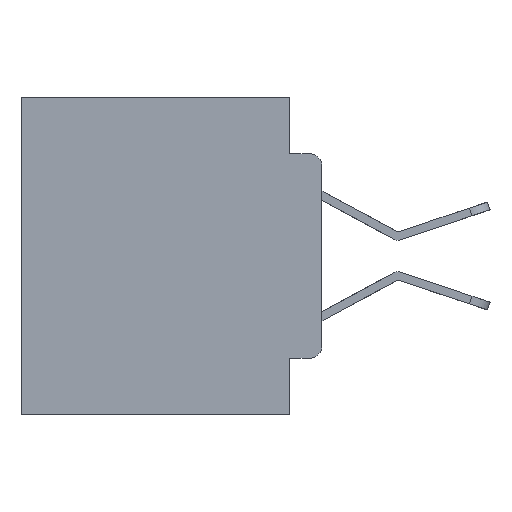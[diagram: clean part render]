
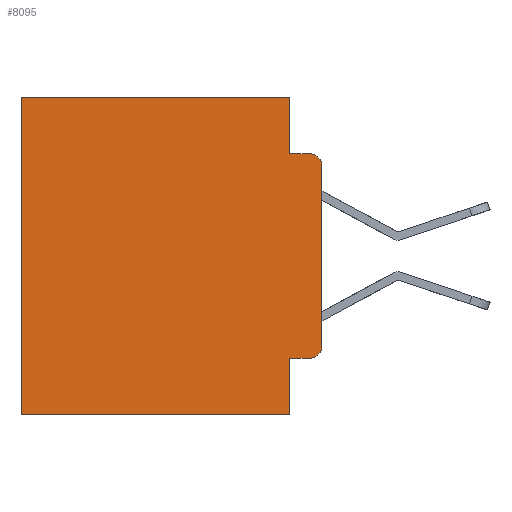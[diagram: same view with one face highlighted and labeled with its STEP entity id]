
A CAD part, left-side view. The second image highlights one B-rep face of the part: STEP entity #8095.
In plain terms, the highlighted planar face has unit normal (-1, 0, 0).
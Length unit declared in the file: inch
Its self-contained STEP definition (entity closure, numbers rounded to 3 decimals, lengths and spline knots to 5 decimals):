
#182 = LINE ( 'NONE', #26400, #10957 ) ;
#1170 = LINE ( 'NONE', #9637, #17663 ) ;
#1172 = AXIS2_PLACEMENT_3D ( 'NONE', #19801, #6941, #21983 ) ;
#1191 = ORIENTED_EDGE ( 'NONE', *, *, #9196, .T. ) ;
#1548 = CARTESIAN_POINT ( 'NONE',  ( 0.298, 0., -0.1085 ) ) ;
#1922 = ORIENTED_EDGE ( 'NONE', *, *, #22513, .T. ) ;
#2360 = CIRCLE ( 'NONE', #20978, 0.02 ) ;
#2890 = LINE ( 'NONE', #6590, #23682 ) ;
#3070 = CARTESIAN_POINT ( 'NONE',  ( 0.298, 0.02, -0.0885 ) ) ;
#3256 = ORIENTED_EDGE ( 'NONE', *, *, #19504, .F. ) ;
#4125 = VERTEX_POINT ( 'NONE', #3070 ) ;
#4140 = DIRECTION ( 'NONE',  ( 0., 0., -1. ) ) ;
#4175 = DIRECTION ( 'NONE',  ( 1., 0., 0. ) ) ;
#4200 = PLANE ( 'NONE',  #6270 ) ;
#4271 = CARTESIAN_POINT ( 'NONE',  ( 0.298, 0., 0. ) ) ;
#4449 = CARTESIAN_POINT ( 'NONE',  ( 0.298, 0., -0.5 ) ) ;
#5339 = LINE ( 'NONE', #4449, #16115 ) ;
#6270 = AXIS2_PLACEMENT_3D ( 'NONE', #4271, #4175, #4140 ) ;
#6590 = CARTESIAN_POINT ( 'NONE',  ( 0.298, 0.051, 0. ) ) ;
#6594 = DIRECTION ( 'NONE',  ( 0., 1., 0. ) ) ;
#6851 = LINE ( 'NONE', #12480, #11910 ) ;
#6941 = DIRECTION ( 'NONE',  ( -1., 0., 0. ) ) ;
#6955 = EDGE_CURVE ( 'NONE', #16703, #4125, #26650, .T. ) ;
#6989 = DIRECTION ( 'NONE',  ( 0., 0., -1. ) ) ;
#7127 = CARTESIAN_POINT ( 'NONE',  ( 0.298, 0.473, -0.5 ) ) ;
#7207 = VERTEX_POINT ( 'NONE', #1548 ) ;
#7759 = DIRECTION ( 'NONE',  ( 0., -1., 0. ) ) ;
#7865 = CARTESIAN_POINT ( 'NONE',  ( 0.298, 0.051, -0.0885 ) ) ;
#7991 = ORIENTED_EDGE ( 'NONE', *, *, #8531, .T. ) ;
#8095 = ADVANCED_FACE ( 'NONE', ( #16720 ), #4200, .F. ) ;
#8531 = EDGE_CURVE ( 'NONE', #12215, #14233, #182, .T. ) ;
#8668 = CARTESIAN_POINT ( 'NONE',  ( 0.298, 0., 0. ) ) ;
#9196 = EDGE_CURVE ( 'NONE', #25642, #13427, #1170, .T. ) ;
#9376 = DIRECTION ( 'NONE',  ( 0., -1., 0. ) ) ;
#9544 = CARTESIAN_POINT ( 'NONE',  ( 0.298, 0.02, -0.1085 ) ) ;
#9637 = CARTESIAN_POINT ( 'NONE',  ( 0.298, 0.473, 0. ) ) ;
#9682 = VECTOR ( 'NONE', #7759, 39.37008 ) ;
#10220 = VECTOR ( 'NONE', #6989, 39.37008 ) ;
#10723 = CARTESIAN_POINT ( 'NONE',  ( 0.298, 0.051, -0.5 ) ) ;
#10957 = VECTOR ( 'NONE', #9376, 39.37008 ) ;
#11684 = DIRECTION ( 'NONE',  ( 0., 0., -1. ) ) ;
#11910 = VECTOR ( 'NONE', #21038, 39.37008 ) ;
#11954 = CARTESIAN_POINT ( 'NONE',  ( 0.298, 0., -0.3915 ) ) ;
#12215 = VERTEX_POINT ( 'NONE', #22609 ) ;
#12480 = CARTESIAN_POINT ( 'NONE',  ( 0.298, 0.051, 0. ) ) ;
#12506 = EDGE_LOOP ( 'NONE', ( #21894, #1922, #16373, #13661, #18630, #1191, #26623, #3256, #7991, #26416 ) ) ;
#13203 = EDGE_CURVE ( 'NONE', #21087, #25642, #22472, .T. ) ;
#13208 = EDGE_CURVE ( 'NONE', #22896, #13427, #5339, .T. ) ;
#13385 = CARTESIAN_POINT ( 'NONE',  ( 0.298, 0.051, 0. ) ) ;
#13427 = VERTEX_POINT ( 'NONE', #7127 ) ;
#13513 = CARTESIAN_POINT ( 'NONE',  ( 0.298, 0., 0. ) ) ;
#13661 = ORIENTED_EDGE ( 'NONE', *, *, #15697, .F. ) ;
#14233 = VERTEX_POINT ( 'NONE', #22978 ) ;
#14571 = CARTESIAN_POINT ( 'NONE',  ( 0.298, 0.051, -0.0885 ) ) ;
#15188 = DIRECTION ( 'NONE',  ( 0., 1., 0. ) ) ;
#15697 = EDGE_CURVE ( 'NONE', #21087, #16703, #2890, .T. ) ;
#16115 = VECTOR ( 'NONE', #6594, 39.37008 ) ;
#16373 = ORIENTED_EDGE ( 'NONE', *, *, #6955, .F. ) ;
#16703 = VERTEX_POINT ( 'NONE', #14571 ) ;
#16720 = FACE_OUTER_BOUND ( 'NONE', #12506, .T. ) ;
#17323 = DIRECTION ( 'NONE',  ( 0., 0., -1. ) ) ;
#17663 = VECTOR ( 'NONE', #18260, 39.37008 ) ;
#18260 = DIRECTION ( 'NONE',  ( 0., 0., -1. ) ) ;
#18630 = ORIENTED_EDGE ( 'NONE', *, *, #13203, .T. ) ;
#19504 = EDGE_CURVE ( 'NONE', #12215, #22896, #6851, .T. ) ;
#19801 = CARTESIAN_POINT ( 'NONE',  ( 0.298, 0.02, -0.3915 ) ) ;
#19859 = EDGE_CURVE ( 'NONE', #7207, #25586, #20977, .T. ) ;
#20568 = CIRCLE ( 'NONE', #1172, 0.02 ) ;
#20977 = LINE ( 'NONE', #13513, #10220 ) ;
#20978 = AXIS2_PLACEMENT_3D ( 'NONE', #9544, #24473, #11684 ) ;
#21038 = DIRECTION ( 'NONE',  ( 0., 0., -1. ) ) ;
#21087 = VERTEX_POINT ( 'NONE', #13385 ) ;
#21894 = ORIENTED_EDGE ( 'NONE', *, *, #19859, .F. ) ;
#21983 = DIRECTION ( 'NONE',  ( 0., 0., -1. ) ) ;
#22472 = LINE ( 'NONE', #8668, #27348 ) ;
#22513 = EDGE_CURVE ( 'NONE', #7207, #4125, #2360, .T. ) ;
#22609 = CARTESIAN_POINT ( 'NONE',  ( 0.298, 0.051, -0.4115 ) ) ;
#22896 = VERTEX_POINT ( 'NONE', #10723 ) ;
#22978 = CARTESIAN_POINT ( 'NONE',  ( 0.298, 0.02, -0.4115 ) ) ;
#23052 = EDGE_CURVE ( 'NONE', #14233, #25586, #20568, .T. ) ;
#23682 = VECTOR ( 'NONE', #17323, 39.37008 ) ;
#24473 = DIRECTION ( 'NONE',  ( -1., 0., 0. ) ) ;
#25586 = VERTEX_POINT ( 'NONE', #11954 ) ;
#25642 = VERTEX_POINT ( 'NONE', #27001 ) ;
#26400 = CARTESIAN_POINT ( 'NONE',  ( 0.298, 0.051, -0.4115 ) ) ;
#26416 = ORIENTED_EDGE ( 'NONE', *, *, #23052, .T. ) ;
#26623 = ORIENTED_EDGE ( 'NONE', *, *, #13208, .F. ) ;
#26650 = LINE ( 'NONE', #7865, #9682 ) ;
#27001 = CARTESIAN_POINT ( 'NONE',  ( 0.298, 0.473, 0. ) ) ;
#27348 = VECTOR ( 'NONE', #15188, 39.37008 ) ;
